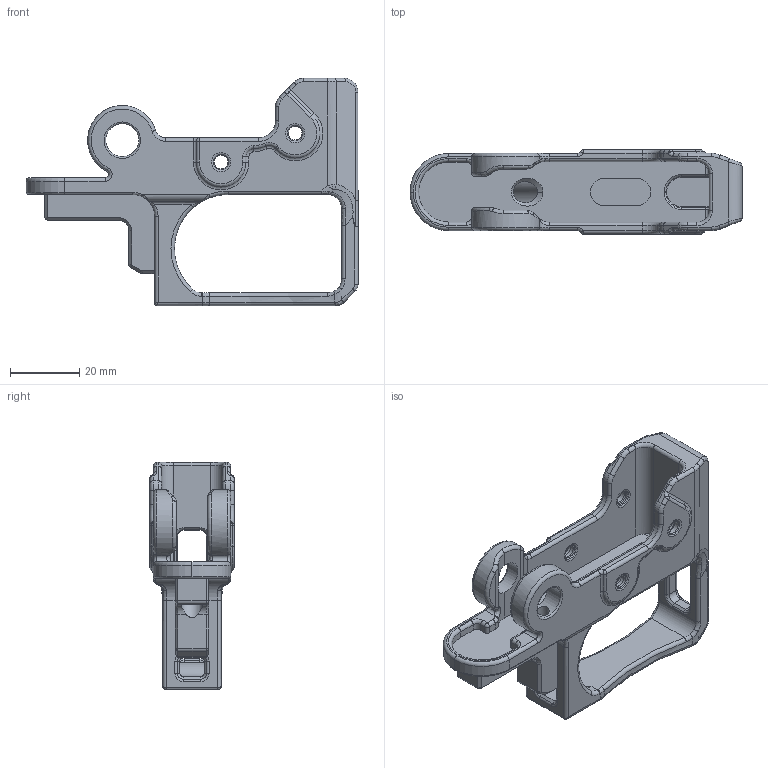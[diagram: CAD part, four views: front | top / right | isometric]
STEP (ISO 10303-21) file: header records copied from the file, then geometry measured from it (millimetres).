
FILE_DESCRIPTION(/* description */ (''),/* implementation_level */ '2;1');
FILE_NAME(/* name */ 'Reduced Material Design.step',/* time_stamp */ '2021-04-08T20:13:17-04:00',/* author */ (''),/* organization */ (''),/* preprocessor_version */ 'ST-DEVELOPER v18.1',/* originating_system */ 'Autodesk Translation Framework v10.6.0.1341',/* authorisation */ '');
FILE_SCHEMA (('AUTOMOTIVE_DESIGN { 1 0 10303 214 3 1 1 }'));
Length unit declared in the file: millimetre
Products named in the file (1): Reduced Material Design
Bounding box: 95.95 x 24.33 x 65.72 mm (x, y, z)
Volume: 27807.3 mm3; surface area: 16863.1 mm2
Topology: 1 solids, 1 shells, 556 faces, 1351 edges, 774 vertices
Faces by surface type: cylinder 189, torus 130, bspline 95, plane 93, cone 41, sphere 8
Full cylindrical faces by diameter (mm): 3.962 x4, 4 x4, 6.097 x1, 9.55 x2
Entity records: 18883 total; most frequent: CARTESIAN_POINT 6123, DIRECTION 2728, ORIENTED_EDGE 2678, EDGE_CURVE 1339, AXIS2_PLACEMENT_3D 1120, VERTEX_POINT 774, CIRCLE 628, EDGE_LOOP 571
